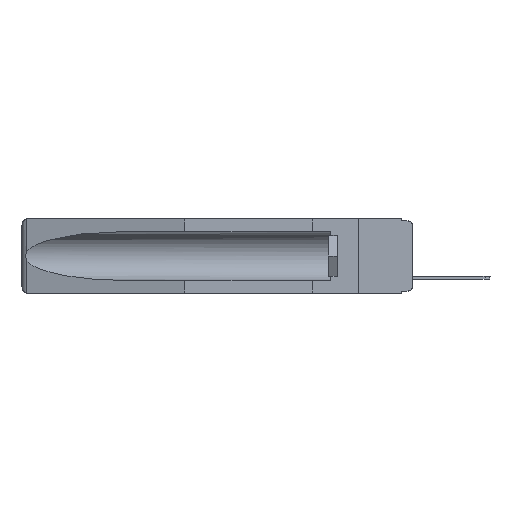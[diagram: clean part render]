
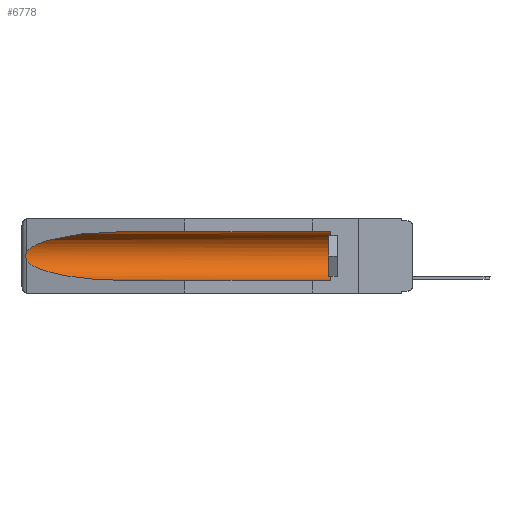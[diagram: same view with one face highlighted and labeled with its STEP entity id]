
A CAD part, left-side view. The second image highlights one B-rep face of the part: STEP entity #6778.
In plain terms, the highlighted cylindrical face has radius 2.857 mm (diameter 5.715 mm), a partial arc.
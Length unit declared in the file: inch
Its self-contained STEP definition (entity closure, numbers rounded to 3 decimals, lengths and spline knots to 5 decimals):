
#888 = ORIENTED_EDGE ( 'NONE', *, *, #16208, .F. ) ;
#950 = CARTESIAN_POINT ( 'NONE',  ( 0.26597, 1.52961, -0.15275 ) ) ;
#1035 = CARTESIAN_POINT ( 'NONE',  ( 0.26654, 1.53092, -0.15636 ) ) ;
#1166 = ORIENTED_EDGE ( 'NONE', *, *, #15620, .T. ) ;
#1327 = EDGE_CURVE ( 'NONE', #14742, #7142, #6384, .T. ) ;
#1459 = LINE ( 'NONE', #6966, #3853 ) ;
#1734 = CARTESIAN_POINT ( 'NONE',  ( 0.25451, 1.48313, -0.24835 ) ) ;
#2055 = ORIENTED_EDGE ( 'NONE', *, *, #11647, .T. ) ;
#2204 = CARTESIAN_POINT ( 'NONE',  ( 0.26597, 1.5296, -0.19026 ) ) ;
#2206 = DIRECTION ( 'NONE',  ( 0., 0., 1. ) ) ;
#2315 = DIRECTION ( 'NONE',  ( 0., 1., 0. ) ) ;
#2600 = CARTESIAN_POINT ( 'NONE',  ( 0.25451, 1.48313, -0.09465 ) ) ;
#2784 = EDGE_CURVE ( 'NONE', #2911, #13546, #7889, .T. ) ;
#2911 = VERTEX_POINT ( 'NONE', #12158 ) ;
#3319 = LINE ( 'NONE', #6229, #14077 ) ;
#3853 = VECTOR ( 'NONE', #5619, 39.37008 ) ;
#4173 = CARTESIAN_POINT ( 'NONE',  ( 0.155, 1.07973, -0.059 ) ) ;
#4710 = DIRECTION ( 'NONE',  ( 0., -1., 0. ) ) ;
#5041 = DIRECTION ( 'NONE',  ( 0., 0., 1. ) ) ;
#5156 = VERTEX_POINT ( 'NONE', #4173 ) ;
#5185 = CARTESIAN_POINT ( 'NONE',  ( 0.2673, 1.5327, -0.16383 ) ) ;
#5409 = CARTESIAN_POINT ( 'NONE',  ( 0.155, 1.07973, -0.059 ) ) ;
#5619 = DIRECTION ( 'NONE',  ( 0., 1., 0. ) ) ;
#5886 = EDGE_CURVE ( 'NONE', #5156, #8024, #17584, .T. ) ;
#6229 = CARTESIAN_POINT ( 'NONE',  ( 0.155, -0.30754, -0.059 ) ) ;
#6384 =( BOUNDED_CURVE ( )  B_SPLINE_CURVE ( 3, ( #15556, #1734, #7331, #7234 ),
 .UNSPECIFIED., .F., .F. ) 
 B_SPLINE_CURVE_WITH_KNOTS ( ( 4, 4 ),
 ( 0.1948, 1.5708 ),
 .UNSPECIFIED. ) 
 CURVE ( )  GEOMETRIC_REPRESENTATION_ITEM ( )  RATIONAL_B_SPLINE_CURVE ( ( 1., 0.848, 0.848, 1. ) ) 
 REPRESENTATION_ITEM ( '' )  );
#6543 = CARTESIAN_POINT ( 'NONE',  ( 0.155, 0.126, -0.059 ) ) ;
#6574 = ORIENTED_EDGE ( 'NONE', *, *, #2784, .T. ) ;
#6778 = ADVANCED_FACE ( 'NONE', ( #12131 ), #12032, .F. ) ;
#6966 = CARTESIAN_POINT ( 'NONE',  ( 0.155, -0.30754, -0.284 ) ) ;
#7142 = VERTEX_POINT ( 'NONE', #9070 ) ;
#7234 = CARTESIAN_POINT ( 'NONE',  ( 0.155, 1.07973, -0.284 ) ) ;
#7331 = CARTESIAN_POINT ( 'NONE',  ( 0.21114, 1.30732, -0.284 ) ) ;
#7611 = CARTESIAN_POINT ( 'NONE',  ( 0.26537, 1.52718, -0.19328 ) ) ;
#7631 = CARTESIAN_POINT ( 'NONE',  ( 0.26537, 1.52718, -0.19328 ) ) ;
#7889 = CIRCLE ( 'NONE', #14815, 0.1125 ) ;
#8024 = VERTEX_POINT ( 'NONE', #15049 ) ;
#8212 = CARTESIAN_POINT ( 'NONE',  ( 0.21114, 1.30732, -0.059 ) ) ;
#8935 = AXIS2_PLACEMENT_3D ( 'NONE', #14769, #16236, #2206 ) ;
#9070 = CARTESIAN_POINT ( 'NONE',  ( 0.155, 1.07973, -0.284 ) ) ;
#9261 = CARTESIAN_POINT ( 'NONE',  ( 0.2675, 1.53308, -0.17534 ) ) ;
#9351 = CARTESIAN_POINT ( 'NONE',  ( 0.26655, 1.53094, -0.18657 ) ) ;
#9390 = CARTESIAN_POINT ( 'NONE',  ( 0.26537, 1.52718, -0.14972 ) ) ;
#11647 = EDGE_CURVE ( 'NONE', #13546, #5156, #3319, .T. ) ;
#11884 = CARTESIAN_POINT ( 'NONE',  ( 0.155, 0.126, -0.1715 ) ) ;
#12032 = CYLINDRICAL_SURFACE ( 'NONE', #8935, 0.1125 ) ;
#12131 = FACE_OUTER_BOUND ( 'NONE', #16181, .T. ) ;
#12158 = CARTESIAN_POINT ( 'NONE',  ( 0.155, 0.126, -0.284 ) ) ;
#13546 = VERTEX_POINT ( 'NONE', #6543 ) ;
#13762 = B_SPLINE_CURVE_WITH_KNOTS ( 'NONE', 3,
 ( #15968, #950, #1035, #5185, #15878, #9261, #17491, #9351, #2204, #7631 ),
 .UNSPECIFIED., .F., .F.,
 ( 4, 2, 2, 2, 4 ),
 ( 0., 0.00029, 0.00058, 0.00087, 0.00117 ),
 .UNSPECIFIED. ) ;
#14073 = ORIENTED_EDGE ( 'NONE', *, *, #1327, .T. ) ;
#14077 = VECTOR ( 'NONE', #2315, 39.37008 ) ;
#14742 = VERTEX_POINT ( 'NONE', #7611 ) ;
#14769 = CARTESIAN_POINT ( 'NONE',  ( 0.155, -0.30754, -0.1715 ) ) ;
#14815 = AXIS2_PLACEMENT_3D ( 'NONE', #11884, #4710, #5041 ) ;
#15049 = CARTESIAN_POINT ( 'NONE',  ( 0.26537, 1.52718, -0.14972 ) ) ;
#15556 = CARTESIAN_POINT ( 'NONE',  ( 0.26537, 1.52718, -0.19328 ) ) ;
#15620 = EDGE_CURVE ( 'NONE', #8024, #14742, #13762, .T. ) ;
#15878 = CARTESIAN_POINT ( 'NONE',  ( 0.2675, 1.53308, -0.16763 ) ) ;
#15968 = CARTESIAN_POINT ( 'NONE',  ( 0.26537, 1.52718, -0.14972 ) ) ;
#16106 = ORIENTED_EDGE ( 'NONE', *, *, #5886, .T. ) ;
#16181 = EDGE_LOOP ( 'NONE', ( #16106, #1166, #14073, #888, #6574, #2055 ) ) ;
#16208 = EDGE_CURVE ( 'NONE', #2911, #7142, #1459, .T. ) ;
#16236 = DIRECTION ( 'NONE',  ( 0., 1., 0. ) ) ;
#17491 = CARTESIAN_POINT ( 'NONE',  ( 0.2673, 1.53269, -0.17917 ) ) ;
#17584 =( BOUNDED_CURVE ( )  B_SPLINE_CURVE ( 3, ( #5409, #8212, #2600, #9390 ),
 .UNSPECIFIED., .F., .F. ) 
 B_SPLINE_CURVE_WITH_KNOTS ( ( 4, 4 ),
 ( 4.71239, 6.08839 ),
 .UNSPECIFIED. ) 
 CURVE ( )  GEOMETRIC_REPRESENTATION_ITEM ( )  RATIONAL_B_SPLINE_CURVE ( ( 1., 0.848, 0.848, 1. ) ) 
 REPRESENTATION_ITEM ( '' )  );
